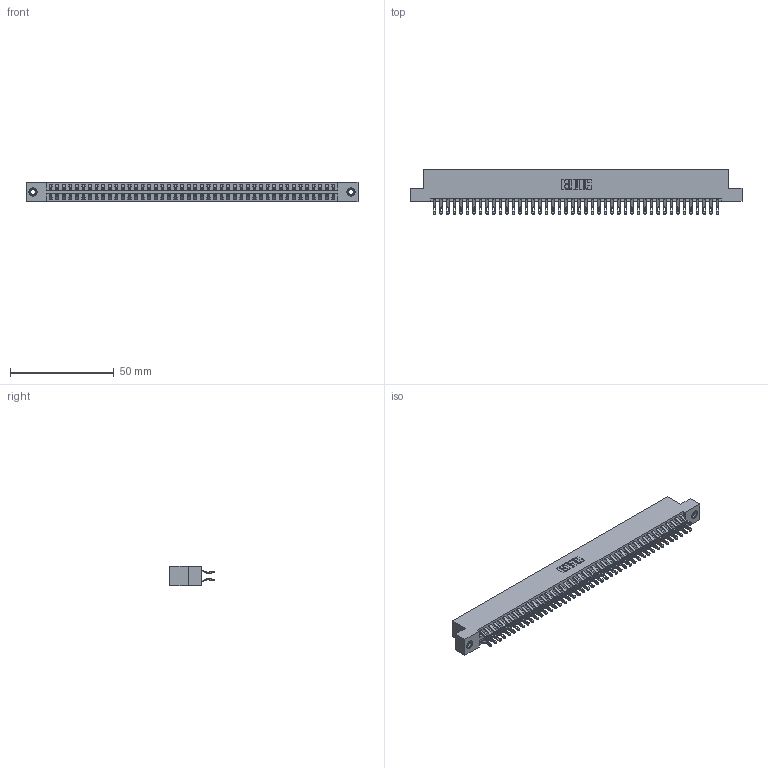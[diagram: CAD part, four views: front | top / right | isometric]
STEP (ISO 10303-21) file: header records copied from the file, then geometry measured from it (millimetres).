
FILE_DESCRIPTION (( 'STEP AP203' ), '1' );
FILE_NAME ('346-088-555-207.STEP', '2022-05-26T01:36:40', ( '' ), ( '' ), 'SwSTEP 2.0', 'SolidWorks 2020', '' );
FILE_SCHEMA (( 'CONFIG_CONTROL_DESIGN' ));
Length unit declared in the file: inch
Products named in the file (4): 345-292-001_555 Tail; 345-250-001_345-250-005-103; 346-088-555-207; 346 Part_Flush Mounting Lugs - 0.156 Dia-TI
Assembly tree (91 placements, depth 2):
  346-088-555-207
    346 Part_Flush Mounting Lugs - 0.156 Dia-TI
    345-292-001_555 Tail  x88
    345-250-001_345-250-005-103  x2
Bounding box: 160.27 x 21.46 x 9.4 mm (x, y, z)
Volume: 15886 mm3; surface area: 22811.4 mm2
Topology: 91 solids, 91 shells, 5286 faces, 16569 edges, 11038 vertices
Faces by surface type: plane 3012, cylinder 2258, cone 12, torus 4
Entity records: 29958 total; most frequent: CARTESIAN_POINT 4953, ORIENTED_EDGE 4850, DIRECTION 4411, EDGE_CURVE 2425, LINE 2077, VECTOR 2077, VERTEX_POINT 1612, AXIS2_PLACEMENT_3D 1167
